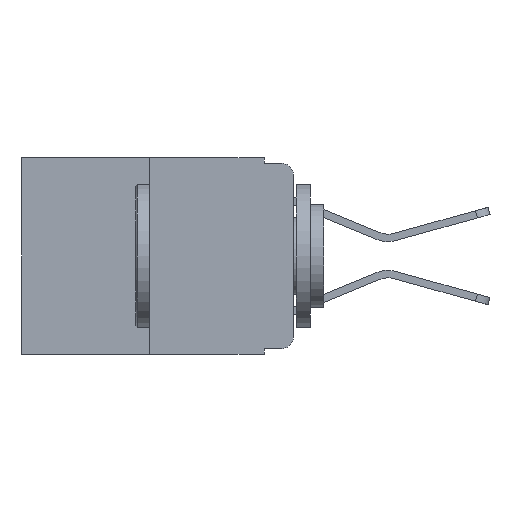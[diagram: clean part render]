
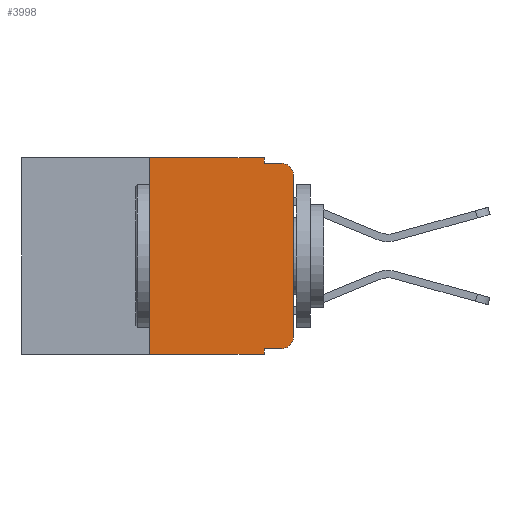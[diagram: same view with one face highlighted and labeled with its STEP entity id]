
A CAD part, left-side view. The second image highlights one B-rep face of the part: STEP entity #3998.
In plain terms, the highlighted planar face has unit normal (-1, 0, 0).
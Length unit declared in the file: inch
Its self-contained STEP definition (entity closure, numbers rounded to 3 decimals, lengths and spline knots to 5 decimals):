
#323 = ORIENTED_EDGE ( 'NONE', *, *, #1848, .F. ) ;
#389 = ORIENTED_EDGE ( 'NONE', *, *, #1898, .T. ) ;
#446 = ORIENTED_EDGE ( 'NONE', *, *, #16308, .F. ) ;
#452 = CARTESIAN_POINT ( 'NONE',  ( 0., 0.051, 0. ) ) ;
#627 = DIRECTION ( 'NONE',  ( 0., -1., 0. ) ) ;
#738 = CARTESIAN_POINT ( 'NONE',  ( 0., 0.473, 0. ) ) ;
#925 = LINE ( 'NONE', #9145, #3263 ) ;
#1544 = VERTEX_POINT ( 'NONE', #16485 ) ;
#1848 = EDGE_CURVE ( 'NONE', #17711, #20449, #4844, .T. ) ;
#1898 = EDGE_CURVE ( 'NONE', #2273, #15987, #1942, .T. ) ;
#1942 = CIRCLE ( 'NONE', #11695, 0.02 ) ;
#1962 = ORIENTED_EDGE ( 'NONE', *, *, #18034, .F. ) ;
#2069 = VERTEX_POINT ( 'NONE', #3558 ) ;
#2273 = VERTEX_POINT ( 'NONE', #15993 ) ;
#2434 = LINE ( 'NONE', #738, #3726 ) ;
#2471 = LINE ( 'NONE', #452, #2910 ) ;
#2653 = CARTESIAN_POINT ( 'NONE',  ( 0., 0.473, 0. ) ) ;
#2910 = VECTOR ( 'NONE', #18542, 39.37008 ) ;
#2996 = VECTOR ( 'NONE', #18312, 39.37008 ) ;
#3157 = EDGE_LOOP ( 'NONE', ( #17339, #12444, #446, #15181, #1962, #323, #9473, #5442, #14839, #389 ) ) ;
#3263 = VECTOR ( 'NONE', #12117, 39.37008 ) ;
#3558 = CARTESIAN_POINT ( 'NONE',  ( 0., 0.051, -0.343 ) ) ;
#3726 = VECTOR ( 'NONE', #627, 39.37008 ) ;
#3989 = LINE ( 'NONE', #10439, #15221 ) ;
#3998 = ADVANCED_FACE ( 'NONE', ( #17331 ), #19042, .F. ) ;
#4153 = VERTEX_POINT ( 'NONE', #12988 ) ;
#4230 = EDGE_CURVE ( 'NONE', #6455, #4153, #10211, .T. ) ;
#4643 = VECTOR ( 'NONE', #16397, 39.37008 ) ;
#4844 = LINE ( 'NONE', #11282, #10706 ) ;
#5202 = CARTESIAN_POINT ( 'NONE',  ( 0., 0., 0. ) ) ;
#5388 = LINE ( 'NONE', #11827, #2996 ) ;
#5442 = ORIENTED_EDGE ( 'NONE', *, *, #12093, .F. ) ;
#6455 = VERTEX_POINT ( 'NONE', #6868 ) ;
#6868 = CARTESIAN_POINT ( 'NONE',  ( 0., 0.051, 0. ) ) ;
#6882 = VERTEX_POINT ( 'NONE', #20005 ) ;
#8098 = DIRECTION ( 'NONE',  ( 0., 0., 1. ) ) ;
#8120 = CARTESIAN_POINT ( 'NONE',  ( 0., 0.02, -0.03 ) ) ;
#8835 = CARTESIAN_POINT ( 'NONE',  ( 0., 0.051, 0. ) ) ;
#8856 = EDGE_CURVE ( 'NONE', #1544, #14001, #10902, .T. ) ;
#8943 = DIRECTION ( 'NONE',  ( 0., -1., 0. ) ) ;
#9145 = CARTESIAN_POINT ( 'NONE',  ( 0., 0.051, -0.333 ) ) ;
#9388 = DIRECTION ( 'NONE',  ( 0., 0., -1. ) ) ;
#9473 = ORIENTED_EDGE ( 'NONE', *, *, #19066, .T. ) ;
#9586 = DIRECTION ( 'NONE',  ( -1., 0., 0. ) ) ;
#9804 = CARTESIAN_POINT ( 'NONE',  ( 0., 0.02, -0.313 ) ) ;
#10047 = LINE ( 'NONE', #5202, #4643 ) ;
#10211 = LINE ( 'NONE', #8835, #10549 ) ;
#10439 = CARTESIAN_POINT ( 'NONE',  ( 0., 0.473, -0.343 ) ) ;
#10549 = VECTOR ( 'NONE', #16459, 39.37008 ) ;
#10659 = DIRECTION ( 'NONE',  ( 1., 0., 0. ) ) ;
#10706 = VECTOR ( 'NONE', #8098, 39.37008 ) ;
#10902 = CIRCLE ( 'NONE', #13942, 0.02 ) ;
#11282 = CARTESIAN_POINT ( 'NONE',  ( 0., 0.25, 0. ) ) ;
#11695 = AXIS2_PLACEMENT_3D ( 'NONE', #9804, #9586, #9388 ) ;
#11827 = CARTESIAN_POINT ( 'NONE',  ( 0., 0.051, -0.01 ) ) ;
#12093 = EDGE_CURVE ( 'NONE', #6882, #2069, #2471, .T. ) ;
#12117 = DIRECTION ( 'NONE',  ( 0., -1., 0. ) ) ;
#12247 = CARTESIAN_POINT ( 'NONE',  ( 0., 0.02, -0.01 ) ) ;
#12444 = ORIENTED_EDGE ( 'NONE', *, *, #8856, .T. ) ;
#12699 = DIRECTION ( 'NONE',  ( -1., 0., 0. ) ) ;
#12988 = CARTESIAN_POINT ( 'NONE',  ( 0., 0.051, -0.01 ) ) ;
#13099 = EDGE_CURVE ( 'NONE', #6882, #2273, #925, .T. ) ;
#13942 = AXIS2_PLACEMENT_3D ( 'NONE', #8120, #12699, #14585 ) ;
#14001 = VERTEX_POINT ( 'NONE', #12247 ) ;
#14585 = DIRECTION ( 'NONE',  ( 0., 0., -1. ) ) ;
#14839 = ORIENTED_EDGE ( 'NONE', *, *, #13099, .T. ) ;
#15149 = EDGE_CURVE ( 'NONE', #15987, #1544, #10047, .T. ) ;
#15181 = ORIENTED_EDGE ( 'NONE', *, *, #4230, .F. ) ;
#15221 = VECTOR ( 'NONE', #8943, 39.37008 ) ;
#15533 = DIRECTION ( 'NONE',  ( 0., 0., -1. ) ) ;
#15987 = VERTEX_POINT ( 'NONE', #18971 ) ;
#15993 = CARTESIAN_POINT ( 'NONE',  ( 0., 0.02, -0.333 ) ) ;
#16308 = EDGE_CURVE ( 'NONE', #4153, #14001, #5388, .T. ) ;
#16397 = DIRECTION ( 'NONE',  ( 0., 0., 1. ) ) ;
#16459 = DIRECTION ( 'NONE',  ( 0., 0., -1. ) ) ;
#16485 = CARTESIAN_POINT ( 'NONE',  ( 0., 0., -0.03 ) ) ;
#16566 = AXIS2_PLACEMENT_3D ( 'NONE', #2653, #10659, #15533 ) ;
#16953 = CARTESIAN_POINT ( 'NONE',  ( 0., 0.25, 0. ) ) ;
#17331 = FACE_OUTER_BOUND ( 'NONE', #3157, .T. ) ;
#17339 = ORIENTED_EDGE ( 'NONE', *, *, #15149, .T. ) ;
#17711 = VERTEX_POINT ( 'NONE', #19052 ) ;
#18034 = EDGE_CURVE ( 'NONE', #20449, #6455, #2434, .T. ) ;
#18312 = DIRECTION ( 'NONE',  ( 0., -1., 0. ) ) ;
#18542 = DIRECTION ( 'NONE',  ( 0., 0., -1. ) ) ;
#18971 = CARTESIAN_POINT ( 'NONE',  ( 0., 0., -0.313 ) ) ;
#19042 = PLANE ( 'NONE',  #16566 ) ;
#19052 = CARTESIAN_POINT ( 'NONE',  ( 0., 0.25, -0.343 ) ) ;
#19066 = EDGE_CURVE ( 'NONE', #17711, #2069, #3989, .T. ) ;
#20005 = CARTESIAN_POINT ( 'NONE',  ( 0., 0.051, -0.333 ) ) ;
#20449 = VERTEX_POINT ( 'NONE', #16953 ) ;
